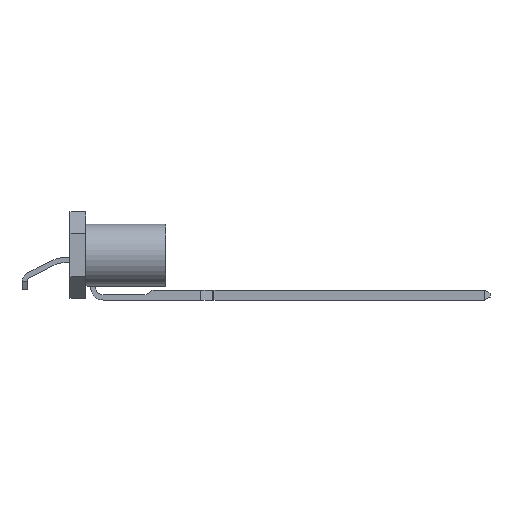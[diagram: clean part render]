
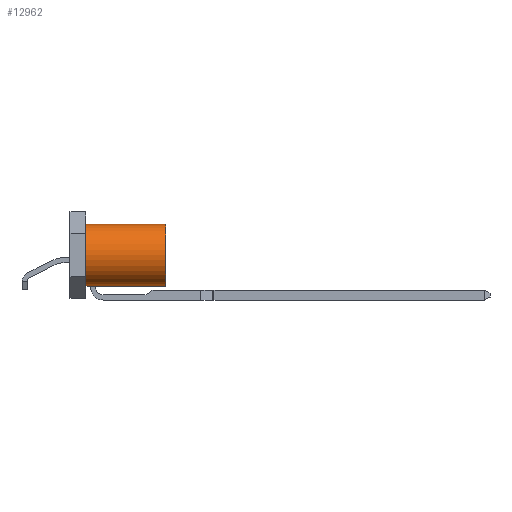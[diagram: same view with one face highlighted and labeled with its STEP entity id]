
A CAD part, left-side view. The second image highlights one B-rep face of the part: STEP entity #12962.
In plain terms, the highlighted cylindrical face has radius 1.968 mm (diameter 3.937 mm), a partial arc.
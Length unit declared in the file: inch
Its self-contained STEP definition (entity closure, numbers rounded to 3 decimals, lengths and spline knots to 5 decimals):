
#916 = CARTESIAN_POINT ( 'NONE',  ( 0., 0.24, -0.0775 ) ) ;
#1407 = CIRCLE ( 'NONE', #12801, 0.0775 ) ;
#2630 = DIRECTION ( 'NONE',  ( 0., -1., 0. ) ) ;
#2698 = CARTESIAN_POINT ( 'NONE',  ( 0., 0.04, 0. ) ) ;
#3976 = EDGE_CURVE ( 'NONE', #11636, #11234, #6368, .T. ) ;
#4216 = CARTESIAN_POINT ( 'NONE',  ( 0., 0.24, 0. ) ) ;
#4289 = DIRECTION ( 'NONE',  ( 0., 0., 1. ) ) ;
#4315 = AXIS2_PLACEMENT_3D ( 'NONE', #2698, #13504, #4289 ) ;
#4889 = EDGE_CURVE ( 'NONE', #11636, #19882, #1407, .T. ) ;
#5037 = ORIENTED_EDGE ( 'NONE', *, *, #6765, .T. ) ;
#6368 = LINE ( 'NONE', #12008, #14079 ) ;
#6405 = VECTOR ( 'NONE', #19392, 39.37008 ) ;
#6765 = EDGE_CURVE ( 'NONE', #11234, #11259, #12129, .T. ) ;
#7011 = EDGE_LOOP ( 'NONE', ( #11328, #7689, #16313, #5037 ) ) ;
#7689 = ORIENTED_EDGE ( 'NONE', *, *, #4889, .F. ) ;
#8727 = CARTESIAN_POINT ( 'NONE',  ( 0., 0.24, 0.0775 ) ) ;
#9072 = DIRECTION ( 'NONE',  ( 0., 1., 0. ) ) ;
#10537 = LINE ( 'NONE', #8727, #6405 ) ;
#10577 = CYLINDRICAL_SURFACE ( 'NONE', #15586, 0.0775 ) ;
#11234 = VERTEX_POINT ( 'NONE', #16984 ) ;
#11259 = VERTEX_POINT ( 'NONE', #15503 ) ;
#11328 = ORIENTED_EDGE ( 'NONE', *, *, #13801, .F. ) ;
#11636 = VERTEX_POINT ( 'NONE', #916 ) ;
#12008 = CARTESIAN_POINT ( 'NONE',  ( 0., 0.24, -0.0775 ) ) ;
#12129 = CIRCLE ( 'NONE', #4315, 0.0775 ) ;
#12440 = CARTESIAN_POINT ( 'NONE',  ( 0., 0.24, 0.0775 ) ) ;
#12801 = AXIS2_PLACEMENT_3D ( 'NONE', #18198, #9072, #19708 ) ;
#12962 = ADVANCED_FACE ( 'NONE', ( #15594 ), #10577, .T. ) ;
#13504 = DIRECTION ( 'NONE',  ( 0., 1., 0. ) ) ;
#13527 = DIRECTION ( 'NONE',  ( 0., -1., 0. ) ) ;
#13801 = EDGE_CURVE ( 'NONE', #19882, #11259, #10537, .T. ) ;
#14079 = VECTOR ( 'NONE', #13527, 39.37008 ) ;
#14931 = DIRECTION ( 'NONE',  ( 0., 0., -1. ) ) ;
#15503 = CARTESIAN_POINT ( 'NONE',  ( 0., 0.04, 0.0775 ) ) ;
#15586 = AXIS2_PLACEMENT_3D ( 'NONE', #4216, #2630, #14931 ) ;
#15594 = FACE_OUTER_BOUND ( 'NONE', #7011, .T. ) ;
#16313 = ORIENTED_EDGE ( 'NONE', *, *, #3976, .T. ) ;
#16984 = CARTESIAN_POINT ( 'NONE',  ( 0., 0.04, -0.0775 ) ) ;
#18198 = CARTESIAN_POINT ( 'NONE',  ( 0., 0.24, 0. ) ) ;
#19392 = DIRECTION ( 'NONE',  ( 0., -1., 0. ) ) ;
#19708 = DIRECTION ( 'NONE',  ( 0., 0., 1. ) ) ;
#19882 = VERTEX_POINT ( 'NONE', #12440 ) ;
